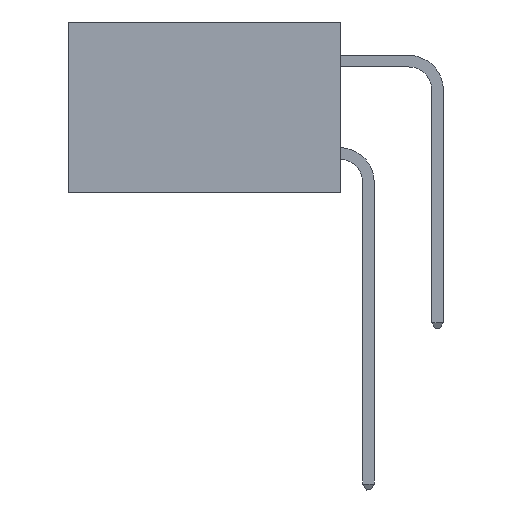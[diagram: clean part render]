
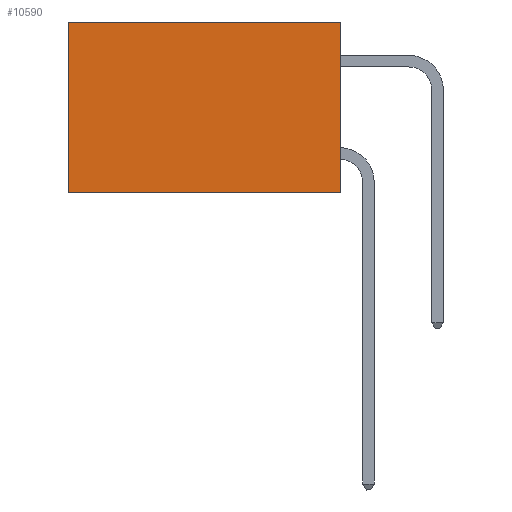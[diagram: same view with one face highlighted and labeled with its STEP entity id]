
A CAD part, left-side view. The second image highlights one B-rep face of the part: STEP entity #10590.
In plain terms, the highlighted planar face has unit normal (-1, 0, 0).
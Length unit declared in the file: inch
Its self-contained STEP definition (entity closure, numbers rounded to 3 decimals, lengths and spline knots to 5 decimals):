
#1234 = CARTESIAN_POINT ( 'NONE',  ( 0.277, 0., -0.37 ) ) ;
#1618 = FACE_OUTER_BOUND ( 'NONE', #28878, .T. ) ;
#2124 = VERTEX_POINT ( 'NONE', #27961 ) ;
#3197 = VERTEX_POINT ( 'NONE', #26232 ) ;
#3898 = LINE ( 'NONE', #1234, #15849 ) ;
#5121 = DIRECTION ( 'NONE',  ( 0., 0., -1. ) ) ;
#5229 = DIRECTION ( 'NONE',  ( 1., 0., 0. ) ) ;
#5328 = CARTESIAN_POINT ( 'NONE',  ( 0.277, 0., -0.37 ) ) ;
#5403 = DIRECTION ( 'NONE',  ( 0., 1., 0. ) ) ;
#5405 = PLANE ( 'NONE',  #19174 ) ;
#6065 = DIRECTION ( 'NONE',  ( 0., 0., -1. ) ) ;
#7768 = CARTESIAN_POINT ( 'NONE',  ( 0.277, 0.59, -0.37 ) ) ;
#8781 = LINE ( 'NONE', #17250, #15826 ) ;
#9418 = LINE ( 'NONE', #28271, #14239 ) ;
#10188 = DIRECTION ( 'NONE',  ( 0., 0., -1. ) ) ;
#10590 = ADVANCED_FACE ( 'NONE', ( #1618 ), #5405, .F. ) ;
#11672 = VECTOR ( 'NONE', #10188, 39.37008 ) ;
#12253 = EDGE_CURVE ( 'NONE', #21736, #25556, #30220, .T. ) ;
#14239 = VECTOR ( 'NONE', #21273, 39.37008 ) ;
#15122 = CARTESIAN_POINT ( 'NONE',  ( 0.277, 0.59, -0.37 ) ) ;
#15826 = VECTOR ( 'NONE', #5403, 39.37008 ) ;
#15834 = ORIENTED_EDGE ( 'NONE', *, *, #12253, .T. ) ;
#15849 = VECTOR ( 'NONE', #6065, 39.37008 ) ;
#17250 = CARTESIAN_POINT ( 'NONE',  ( 0.277, 0., 0. ) ) ;
#17672 = ORIENTED_EDGE ( 'NONE', *, *, #22863, .T. ) ;
#17834 = CARTESIAN_POINT ( 'NONE',  ( 0.277, 0.59, 0. ) ) ;
#19174 = AXIS2_PLACEMENT_3D ( 'NONE', #5328, #5229, #5121 ) ;
#21273 = DIRECTION ( 'NONE',  ( 0., 1., 0. ) ) ;
#21736 = VERTEX_POINT ( 'NONE', #17834 ) ;
#22375 = EDGE_CURVE ( 'NONE', #2124, #3197, #3898, .T. ) ;
#22863 = EDGE_CURVE ( 'NONE', #2124, #21736, #8781, .T. ) ;
#24639 = EDGE_CURVE ( 'NONE', #3197, #25556, #9418, .T. ) ;
#24811 = ORIENTED_EDGE ( 'NONE', *, *, #24639, .F. ) ;
#25556 = VERTEX_POINT ( 'NONE', #15122 ) ;
#26232 = CARTESIAN_POINT ( 'NONE',  ( 0.277, 0., -0.37 ) ) ;
#27961 = CARTESIAN_POINT ( 'NONE',  ( 0.277, 0., 0. ) ) ;
#28271 = CARTESIAN_POINT ( 'NONE',  ( 0.277, 0., -0.37 ) ) ;
#28878 = EDGE_LOOP ( 'NONE', ( #15834, #24811, #28991, #17672 ) ) ;
#28991 = ORIENTED_EDGE ( 'NONE', *, *, #22375, .F. ) ;
#30220 = LINE ( 'NONE', #7768, #11672 ) ;
